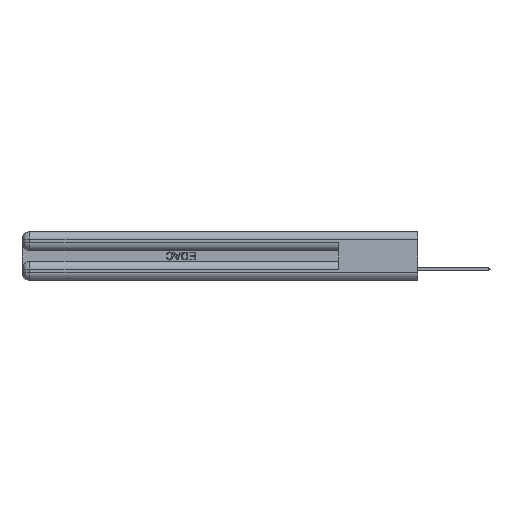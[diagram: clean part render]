
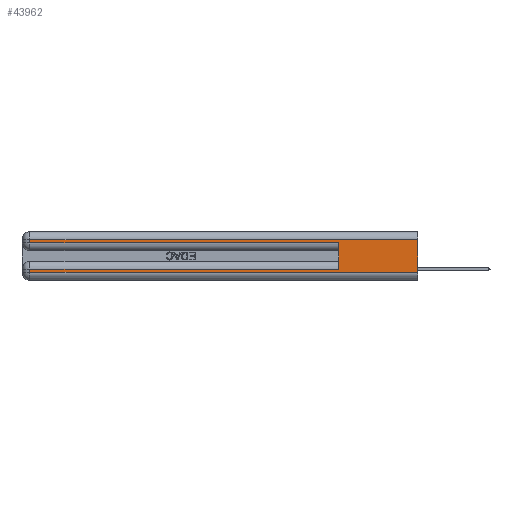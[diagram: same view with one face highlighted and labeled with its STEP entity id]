
A CAD part, left-side view. The second image highlights one B-rep face of the part: STEP entity #43962.
In plain terms, the highlighted planar face has unit normal (-1, 0, 0).
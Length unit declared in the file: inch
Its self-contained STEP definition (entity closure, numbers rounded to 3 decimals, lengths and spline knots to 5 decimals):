
#940 = EDGE_CURVE ( 'NONE', #45903, #12357, #9570, .T. ) ;
#1956 = CARTESIAN_POINT ( 'NONE',  ( 0., 0., 0.085 ) ) ;
#2436 = CARTESIAN_POINT ( 'NONE',  ( 0., 0., 0.31 ) ) ;
#3033 = EDGE_CURVE ( 'NONE', #24200, #13177, #30892, .T. ) ;
#3261 = DIRECTION ( 'NONE',  ( 0., -1., 0. ) ) ;
#5120 = EDGE_CURVE ( 'NONE', #43942, #49615, #28668, .T. ) ;
#6664 = ORIENTED_EDGE ( 'NONE', *, *, #29826, .T. ) ;
#8797 = VERTEX_POINT ( 'NONE', #51418 ) ;
#9570 = LINE ( 'NONE', #17092, #42438 ) ;
#10604 = EDGE_CURVE ( 'NONE', #8797, #12357, #43946, .T. ) ;
#11031 = CARTESIAN_POINT ( 'NONE',  ( 0., 0.6, 0.285 ) ) ;
#12010 = CARTESIAN_POINT ( 'NONE',  ( 0., 0.6, 0.085 ) ) ;
#12033 = DIRECTION ( 'NONE',  ( 0., 0., 1. ) ) ;
#12357 = VERTEX_POINT ( 'NONE', #11031 ) ;
#12806 = VECTOR ( 'NONE', #42022, 39.37008 ) ;
#13177 = VERTEX_POINT ( 'NONE', #18019 ) ;
#14821 = PLANE ( 'NONE',  #48982 ) ;
#15119 = EDGE_CURVE ( 'NONE', #49615, #8797, #27374, .T. ) ;
#15180 = DIRECTION ( 'NONE',  ( 0., 0., -1. ) ) ;
#15963 = CARTESIAN_POINT ( 'NONE',  ( 0., 2.94, 0.31 ) ) ;
#16610 = VECTOR ( 'NONE', #30297, 39.37008 ) ;
#17092 = CARTESIAN_POINT ( 'NONE',  ( 0., 0.6, 0.145 ) ) ;
#17773 = ORIENTED_EDGE ( 'NONE', *, *, #33980, .F. ) ;
#17868 = DIRECTION ( 'NONE',  ( 0., -1., 0. ) ) ;
#18019 = CARTESIAN_POINT ( 'NONE',  ( 0., 0., 0.06 ) ) ;
#18869 = CARTESIAN_POINT ( 'NONE',  ( 0., 0., 0.06 ) ) ;
#19170 = LINE ( 'NONE', #45395, #35487 ) ;
#19514 = CARTESIAN_POINT ( 'NONE',  ( 0., 2.94, 0.06 ) ) ;
#21043 = ORIENTED_EDGE ( 'NONE', *, *, #940, .F. ) ;
#21965 = VECTOR ( 'NONE', #3261, 39.37008 ) ;
#22353 = VECTOR ( 'NONE', #47626, 39.37008 ) ;
#24200 = VERTEX_POINT ( 'NONE', #19514 ) ;
#27374 = LINE ( 'NONE', #29754, #12806 ) ;
#28668 = LINE ( 'NONE', #2436, #22353 ) ;
#29754 = CARTESIAN_POINT ( 'NONE',  ( 0., 2.94, 0.37 ) ) ;
#29826 = EDGE_CURVE ( 'NONE', #45903, #35485, #44528, .T. ) ;
#30297 = DIRECTION ( 'NONE',  ( 0., 1., 0. ) ) ;
#30683 = DIRECTION ( 'NONE',  ( 1., 0., 0. ) ) ;
#30892 = LINE ( 'NONE', #18869, #21965 ) ;
#31327 = ORIENTED_EDGE ( 'NONE', *, *, #5120, .T. ) ;
#32094 = LINE ( 'NONE', #35677, #42828 ) ;
#32206 = ORIENTED_EDGE ( 'NONE', *, *, #10604, .T. ) ;
#33895 = ORIENTED_EDGE ( 'NONE', *, *, #3033, .T. ) ;
#33980 = EDGE_CURVE ( 'NONE', #43942, #13177, #32094, .T. ) ;
#35485 = VERTEX_POINT ( 'NONE', #45520 ) ;
#35487 = VECTOR ( 'NONE', #49775, 39.37008 ) ;
#35677 = CARTESIAN_POINT ( 'NONE',  ( 0., 0., 0.37 ) ) ;
#37225 = FACE_OUTER_BOUND ( 'NONE', #42127, .T. ) ;
#41340 = VECTOR ( 'NONE', #17868, 39.37008 ) ;
#41949 = CARTESIAN_POINT ( 'NONE',  ( 0., 0., 0.285 ) ) ;
#42022 = DIRECTION ( 'NONE',  ( 0., 0., -1. ) ) ;
#42127 = EDGE_LOOP ( 'NONE', ( #17773, #31327, #43796, #32206, #21043, #6664, #44944, #33895 ) ) ;
#42438 = VECTOR ( 'NONE', #12033, 39.37008 ) ;
#42828 = VECTOR ( 'NONE', #43870, 39.37008 ) ;
#43506 = CARTESIAN_POINT ( 'NONE',  ( 0., 0., 0.31 ) ) ;
#43796 = ORIENTED_EDGE ( 'NONE', *, *, #15119, .T. ) ;
#43870 = DIRECTION ( 'NONE',  ( 0., 0., -1. ) ) ;
#43942 = VERTEX_POINT ( 'NONE', #43506 ) ;
#43946 = LINE ( 'NONE', #41949, #41340 ) ;
#43962 = ADVANCED_FACE ( 'NONE', ( #37225 ), #14821, .F. ) ;
#44528 = LINE ( 'NONE', #1956, #16610 ) ;
#44944 = ORIENTED_EDGE ( 'NONE', *, *, #50302, .T. ) ;
#45395 = CARTESIAN_POINT ( 'NONE',  ( 0., 2.94, 0.37 ) ) ;
#45520 = CARTESIAN_POINT ( 'NONE',  ( 0., 2.94, 0.085 ) ) ;
#45903 = VERTEX_POINT ( 'NONE', #12010 ) ;
#47027 = CARTESIAN_POINT ( 'NONE',  ( 0., 0., 0.37 ) ) ;
#47626 = DIRECTION ( 'NONE',  ( 0., 1., 0. ) ) ;
#48982 = AXIS2_PLACEMENT_3D ( 'NONE', #47027, #30683, #15180 ) ;
#49615 = VERTEX_POINT ( 'NONE', #15963 ) ;
#49775 = DIRECTION ( 'NONE',  ( 0., 0., -1. ) ) ;
#50302 = EDGE_CURVE ( 'NONE', #35485, #24200, #19170, .T. ) ;
#51418 = CARTESIAN_POINT ( 'NONE',  ( 0., 2.94, 0.285 ) ) ;
